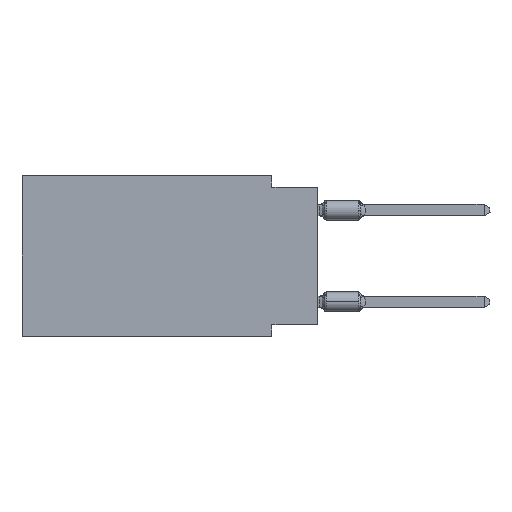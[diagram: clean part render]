
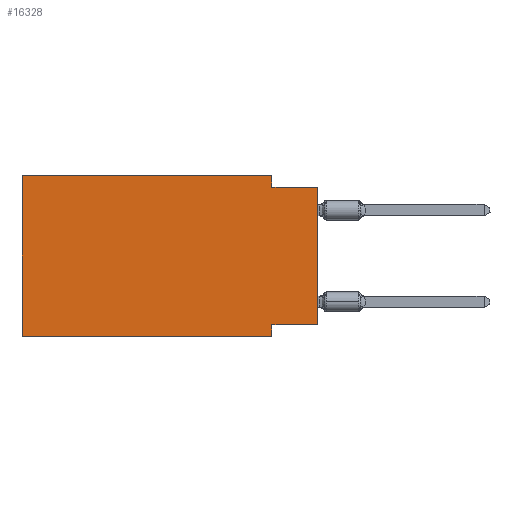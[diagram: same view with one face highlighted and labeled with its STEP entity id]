
A CAD part, left-side view. The second image highlights one B-rep face of the part: STEP entity #16328.
In plain terms, the highlighted planar face has unit normal (-1, 0, 0).
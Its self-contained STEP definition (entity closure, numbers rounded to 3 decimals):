
#232 = AXIS2_PLACEMENT_3D ( 'NONE', #4088, #49712, #3557 ) ;
#1181 = ORIENTED_EDGE ( 'NONE', *, *, #23154, .F. ) ;
#1689 = VERTEX_POINT ( 'NONE', #35379 ) ;
#2038 = VERTEX_POINT ( 'NONE', #14136 ) ;
#2101 = ORIENTED_EDGE ( 'NONE', *, *, #47741, .F. ) ;
#3557 = DIRECTION ( 'NONE',  ( 0., 0., -1. ) ) ;
#4088 = CARTESIAN_POINT ( 'NONE',  ( 0., 16.383, 0. ) ) ;
#4988 = DIRECTION ( 'NONE',  ( 0., 0., 1. ) ) ;
#5195 = VECTOR ( 'NONE', #27204, 1000. ) ;
#6198 = CARTESIAN_POINT ( 'NONE',  ( 0., 2.54, -8.89 ) ) ;
#6869 = LINE ( 'NONE', #47887, #45882 ) ;
#8801 = DIRECTION ( 'NONE',  ( 0., -1., 0. ) ) ;
#9060 = CARTESIAN_POINT ( 'NONE',  ( 0., 16.383, 0. ) ) ;
#9963 = VERTEX_POINT ( 'NONE', #47323 ) ;
#10653 = LINE ( 'NONE', #19323, #5195 ) ;
#10966 = VECTOR ( 'NONE', #4988, 1000. ) ;
#11868 = CARTESIAN_POINT ( 'NONE',  ( 0., 16.383, -8.89 ) ) ;
#11959 = PLANE ( 'NONE',  #232 ) ;
#12062 = ORIENTED_EDGE ( 'NONE', *, *, #49223, .T. ) ;
#12607 = LINE ( 'NONE', #37843, #21188 ) ;
#13882 = VECTOR ( 'NONE', #26479, 1000. ) ;
#14136 = CARTESIAN_POINT ( 'NONE',  ( 0., 0., -8.255 ) ) ;
#15464 = VERTEX_POINT ( 'NONE', #19229 ) ;
#16328 = ADVANCED_FACE ( 'NONE', ( #41554 ), #11959, .F. ) ;
#17385 = VERTEX_POINT ( 'NONE', #46291 ) ;
#17781 = CARTESIAN_POINT ( 'NONE',  ( 0., 16.383, 0. ) ) ;
#18395 = CARTESIAN_POINT ( 'NONE',  ( 0., 0., -8.255 ) ) ;
#19229 = CARTESIAN_POINT ( 'NONE',  ( 0., 0., -0.635 ) ) ;
#19323 = CARTESIAN_POINT ( 'NONE',  ( 0., 0., 0. ) ) ;
#19468 = DIRECTION ( 'NONE',  ( 0., 1., 0. ) ) ;
#21188 = VECTOR ( 'NONE', #8801, 1000. ) ;
#22895 = DIRECTION ( 'NONE',  ( 0., 0., -1. ) ) ;
#23154 = EDGE_CURVE ( 'NONE', #36510, #17385, #29690, .T. ) ;
#24380 = DIRECTION ( 'NONE',  ( 0., -1., 0. ) ) ;
#24619 = CARTESIAN_POINT ( 'NONE',  ( 0., 2.54, -8.255 ) ) ;
#26479 = DIRECTION ( 'NONE',  ( 0., -1., 0. ) ) ;
#26735 = VERTEX_POINT ( 'NONE', #24619 ) ;
#27204 = DIRECTION ( 'NONE',  ( 0., 0., 1. ) ) ;
#27658 = EDGE_CURVE ( 'NONE', #26735, #52174, #6869, .T. ) ;
#28234 = EDGE_CURVE ( 'NONE', #1689, #9963, #29500, .T. ) ;
#28411 = ORIENTED_EDGE ( 'NONE', *, *, #43121, .T. ) ;
#28839 = VECTOR ( 'NONE', #19468, 1000. ) ;
#29500 = LINE ( 'NONE', #36602, #43323 ) ;
#29690 = LINE ( 'NONE', #9060, #10966 ) ;
#30683 = VECTOR ( 'NONE', #24380, 1000. ) ;
#31163 = ORIENTED_EDGE ( 'NONE', *, *, #28234, .F. ) ;
#34777 = EDGE_CURVE ( 'NONE', #17385, #1689, #51226, .T. ) ;
#35379 = CARTESIAN_POINT ( 'NONE',  ( 0., 2.54, 0. ) ) ;
#36510 = VERTEX_POINT ( 'NONE', #44714 ) ;
#36602 = CARTESIAN_POINT ( 'NONE',  ( 0., 2.54, 0. ) ) ;
#37843 = CARTESIAN_POINT ( 'NONE',  ( 0., 0., -0.635 ) ) ;
#41554 = FACE_OUTER_BOUND ( 'NONE', #51748, .T. ) ;
#41775 = ORIENTED_EDGE ( 'NONE', *, *, #49644, .F. ) ;
#43121 = EDGE_CURVE ( 'NONE', #2038, #15464, #10653, .T. ) ;
#43323 = VECTOR ( 'NONE', #46601, 1000. ) ;
#43500 = ORIENTED_EDGE ( 'NONE', *, *, #34777, .F. ) ;
#43658 = LINE ( 'NONE', #18395, #28839 ) ;
#44714 = CARTESIAN_POINT ( 'NONE',  ( 0., 16.383, -8.89 ) ) ;
#45882 = VECTOR ( 'NONE', #22895, 1000. ) ;
#46291 = CARTESIAN_POINT ( 'NONE',  ( 0., 16.383, 0. ) ) ;
#46601 = DIRECTION ( 'NONE',  ( 0., 0., -1. ) ) ;
#47323 = CARTESIAN_POINT ( 'NONE',  ( 0., 2.54, -0.635 ) ) ;
#47741 = EDGE_CURVE ( 'NONE', #2038, #26735, #43658, .T. ) ;
#47787 = ORIENTED_EDGE ( 'NONE', *, *, #27658, .F. ) ;
#47887 = CARTESIAN_POINT ( 'NONE',  ( 0., 2.54, -8.89 ) ) ;
#49081 = LINE ( 'NONE', #11868, #30683 ) ;
#49223 = EDGE_CURVE ( 'NONE', #36510, #52174, #49081, .T. ) ;
#49644 = EDGE_CURVE ( 'NONE', #9963, #15464, #12607, .T. ) ;
#49712 = DIRECTION ( 'NONE',  ( 1., 0., 0. ) ) ;
#51226 = LINE ( 'NONE', #17781, #13882 ) ;
#51748 = EDGE_LOOP ( 'NONE', ( #28411, #41775, #31163, #43500, #1181, #12062, #47787, #2101 ) ) ;
#52174 = VERTEX_POINT ( 'NONE', #6198 ) ;
